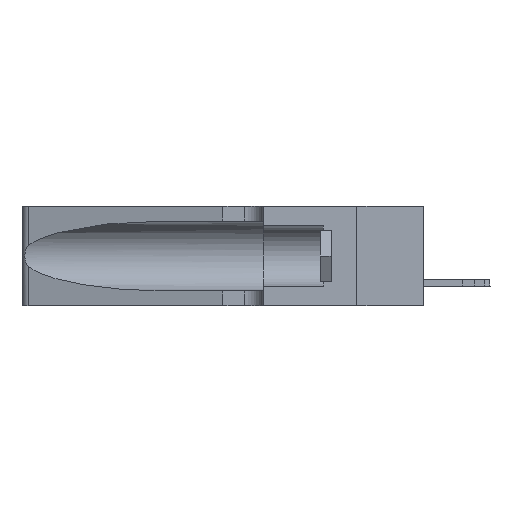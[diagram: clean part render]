
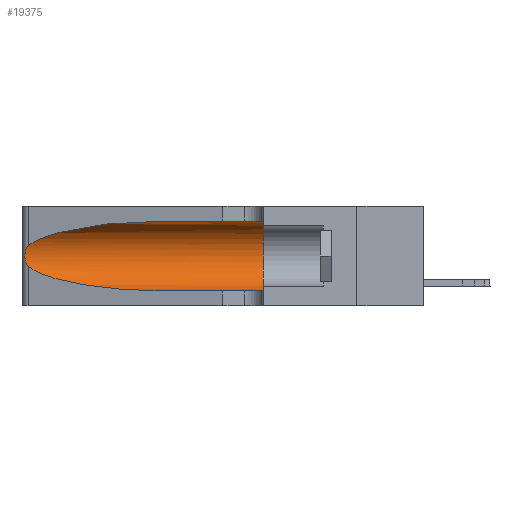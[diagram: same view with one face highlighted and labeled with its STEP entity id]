
A CAD part, left-side view. The second image highlights one B-rep face of the part: STEP entity #19375.
In plain terms, the highlighted cylindrical face has radius 3.308 mm (diameter 6.617 mm), a partial arc.
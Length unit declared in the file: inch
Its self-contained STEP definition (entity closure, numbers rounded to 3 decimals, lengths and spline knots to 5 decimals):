
#767 =( BOUNDED_CURVE ( )  B_SPLINE_CURVE ( 3, ( #17079, #2695, #10151, #17388 ),
 .UNSPECIFIED., .F., .F. ) 
 B_SPLINE_CURVE_WITH_KNOTS ( ( 4, 4 ),
 ( 1.5708, 2.84003 ),
 .UNSPECIFIED. ) 
 CURVE ( )  GEOMETRIC_REPRESENTATION_ITEM ( )  RATIONAL_B_SPLINE_CURVE ( ( 1., 0.87, 0.87, 1. ) ) 
 REPRESENTATION_ITEM ( '' )  );
#994 = EDGE_CURVE ( 'NONE', #4444, #22806, #14497, .T. ) ;
#1288 = LINE ( 'NONE', #3516, #26150 ) ;
#1946 = CARTESIAN_POINT ( 'NONE',  ( 0.25487, 1.22718, 0.22369 ) ) ;
#2203 = AXIS2_PLACEMENT_3D ( 'NONE', #20951, #30998, #23705 ) ;
#2660 = CARTESIAN_POINT ( 'NONE',  ( 0.1305, 1.61858, 0.31525 ) ) ;
#2695 = CARTESIAN_POINT ( 'NONE',  ( 0.18966, 0.96281, 0.31525 ) ) ;
#2805 = EDGE_CURVE ( 'NONE', #22806, #5636, #19483, .T. ) ;
#3011 = FACE_OUTER_BOUND ( 'NONE', #16925, .T. ) ;
#3154 = EDGE_CURVE ( 'NONE', #4444, #11641, #767, .T. ) ;
#3516 = CARTESIAN_POINT ( 'NONE',  ( 0.1305, 1.61858, 0.05475 ) ) ;
#3769 = ORIENTED_EDGE ( 'NONE', *, *, #24160, .T. ) ;
#4444 = VERTEX_POINT ( 'NONE', #6580 ) ;
#4458 = CARTESIAN_POINT ( 'NONE',  ( 0.25789, 1.23486, 0.15765 ) ) ;
#5636 = VERTEX_POINT ( 'NONE', #16273 ) ;
#6361 = VERTEX_POINT ( 'NONE', #15818 ) ;
#6580 = CARTESIAN_POINT ( 'NONE',  ( 0.1305, 0.72297, 0.31525 ) ) ;
#6663 = CARTESIAN_POINT ( 'NONE',  ( 0.26075, 1.23896, 0.178 ) ) ;
#6898 = CARTESIAN_POINT ( 'NONE',  ( 0.25555, 1.22993, 0.14849 ) ) ;
#8374 = DIRECTION ( 'NONE',  ( 0., -1., 0. ) ) ;
#10151 = CARTESIAN_POINT ( 'NONE',  ( 0.2373, 1.15595, 0.28018 ) ) ;
#11247 = CARTESIAN_POINT ( 'NONE',  ( 0.1305, 0.72297, 0.05475 ) ) ;
#11573 = CARTESIAN_POINT ( 'NONE',  ( 0.25787, 1.23484, 0.2124 ) ) ;
#11641 = VERTEX_POINT ( 'NONE', #29964 ) ;
#11816 = DIRECTION ( 'NONE',  ( 0., 1., 0. ) ) ;
#13589 = CYLINDRICAL_SURFACE ( 'NONE', #2203, 0.13025 ) ;
#13686 = ORIENTED_EDGE ( 'NONE', *, *, #3154, .T. ) ;
#14193 = AXIS2_PLACEMENT_3D ( 'NONE', #28918, #11816, #28480 ) ;
#14284 = EDGE_CURVE ( 'NONE', #17938, #5636, #1288, .T. ) ;
#14337 = ORIENTED_EDGE ( 'NONE', *, *, #2805, .F. ) ;
#14385 = EDGE_CURVE ( 'NONE', #6361, #17938, #29654, .T. ) ;
#14497 = LINE ( 'NONE', #2660, #23536 ) ;
#15774 = CARTESIAN_POINT ( 'NONE',  ( 0.18966, 0.96281, 0.05475 ) ) ;
#15818 = CARTESIAN_POINT ( 'NONE',  ( 0.25487, 1.22718, 0.14631 ) ) ;
#16171 = CARTESIAN_POINT ( 'NONE',  ( 0.1305, 0.35, 0.31525 ) ) ;
#16199 = CARTESIAN_POINT ( 'NONE',  ( 0.26075, 1.23896, 0.19203 ) ) ;
#16273 = CARTESIAN_POINT ( 'NONE',  ( 0.1305, 0.35, 0.05475 ) ) ;
#16312 = CARTESIAN_POINT ( 'NONE',  ( 0.25856, 1.23593, 0.16098 ) ) ;
#16418 = CARTESIAN_POINT ( 'NONE',  ( 0.26018, 1.23835, 0.19895 ) ) ;
#16925 = EDGE_LOOP ( 'NONE', ( #13686, #3769, #23057, #25168, #14337, #24265 ) ) ;
#17079 = CARTESIAN_POINT ( 'NONE',  ( 0.1305, 0.72297, 0.31525 ) ) ;
#17388 = CARTESIAN_POINT ( 'NONE',  ( 0.25487, 1.22718, 0.22369 ) ) ;
#17695 = CARTESIAN_POINT ( 'NONE',  ( 0.2373, 1.15595, 0.08982 ) ) ;
#17938 = VERTEX_POINT ( 'NONE', #17984 ) ;
#17984 = CARTESIAN_POINT ( 'NONE',  ( 0.1305, 0.72297, 0.05475 ) ) ;
#18856 = CARTESIAN_POINT ( 'NONE',  ( 0.25555, 1.22994, 0.2215 ) ) ;
#19375 = ADVANCED_FACE ( 'NONE', ( #3011 ), #13589, .F. ) ;
#19483 = CIRCLE ( 'NONE', #14193, 0.13025 ) ;
#20951 = CARTESIAN_POINT ( 'NONE',  ( 0.1305, 1.61858, 0.185 ) ) ;
#21286 = CARTESIAN_POINT ( 'NONE',  ( 0.25487, 1.22718, 0.14631 ) ) ;
#21849 = CARTESIAN_POINT ( 'NONE',  ( 0.25487, 1.22718, 0.14631 ) ) ;
#22806 = VERTEX_POINT ( 'NONE', #16171 ) ;
#23057 = ORIENTED_EDGE ( 'NONE', *, *, #14385, .T. ) ;
#23489 = CARTESIAN_POINT ( 'NONE',  ( 0.26017, 1.23833, 0.17102 ) ) ;
#23536 = VECTOR ( 'NONE', #31112, 39.37008 ) ;
#23705 = DIRECTION ( 'NONE',  ( 0., 0., -1. ) ) ;
#24160 = EDGE_CURVE ( 'NONE', #11641, #6361, #26382, .T. ) ;
#24265 = ORIENTED_EDGE ( 'NONE', *, *, #994, .F. ) ;
#25168 = ORIENTED_EDGE ( 'NONE', *, *, #14284, .T. ) ;
#26150 = VECTOR ( 'NONE', #8374, 39.37008 ) ;
#26245 = CARTESIAN_POINT ( 'NONE',  ( 0.25854, 1.2359, 0.20912 ) ) ;
#26382 = B_SPLINE_CURVE_WITH_KNOTS ( 'NONE', 3,
 ( #1946, #18856, #30999, #11573, #26245, #16418, #16199, #6663, #23489, #16312, #4458, #28569, #6898, #21286 ),
 .UNSPECIFIED., .F., .F.,
 ( 4, 2, 2, 2, 2, 2, 4 ),
 ( 0., 0.00027, 0.00053, 0.00107, 0.0016, 0.00187, 0.00214 ),
 .UNSPECIFIED. ) ;
#28480 = DIRECTION ( 'NONE',  ( 0., 0., 1. ) ) ;
#28569 = CARTESIAN_POINT ( 'NONE',  ( 0.25639, 1.23186, 0.15144 ) ) ;
#28918 = CARTESIAN_POINT ( 'NONE',  ( 0.1305, 0.35, 0.185 ) ) ;
#29654 =( BOUNDED_CURVE ( )  B_SPLINE_CURVE ( 3, ( #21849, #17695, #15774, #11247 ),
 .UNSPECIFIED., .F., .F. ) 
 B_SPLINE_CURVE_WITH_KNOTS ( ( 4, 4 ),
 ( 3.44316, 4.71239 ),
 .UNSPECIFIED. ) 
 CURVE ( )  GEOMETRIC_REPRESENTATION_ITEM ( )  RATIONAL_B_SPLINE_CURVE ( ( 1., 0.87, 0.87, 1. ) ) 
 REPRESENTATION_ITEM ( '' )  );
#29964 = CARTESIAN_POINT ( 'NONE',  ( 0.25487, 1.22718, 0.22369 ) ) ;
#30998 = DIRECTION ( 'NONE',  ( 0., -1., 0. ) ) ;
#30999 = CARTESIAN_POINT ( 'NONE',  ( 0.25639, 1.23184, 0.21858 ) ) ;
#31112 = DIRECTION ( 'NONE',  ( 0., -1., 0. ) ) ;
